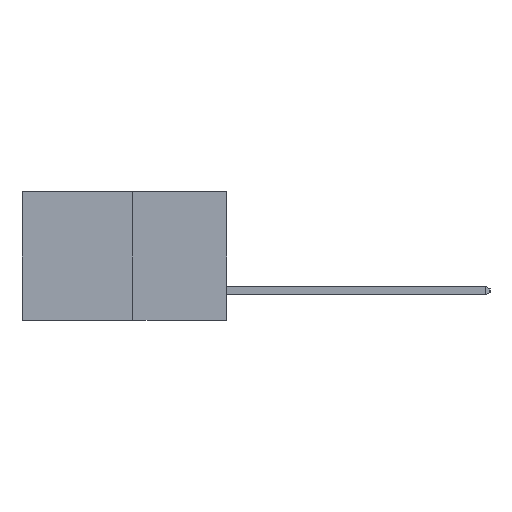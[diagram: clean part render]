
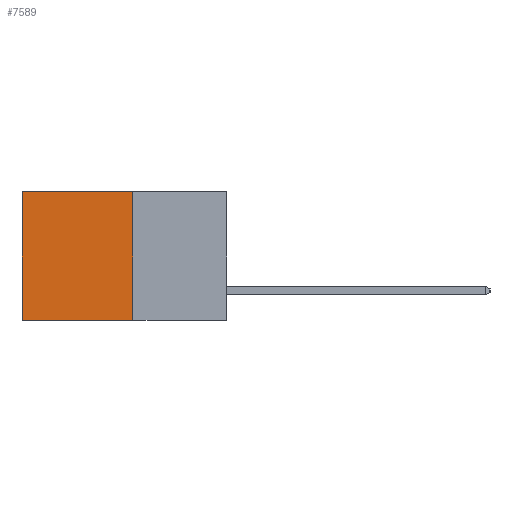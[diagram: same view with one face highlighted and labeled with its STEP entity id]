
A CAD part, left-side view. The second image highlights one B-rep face of the part: STEP entity #7589.
In plain terms, the highlighted planar face has unit normal (-1, 0, 0).
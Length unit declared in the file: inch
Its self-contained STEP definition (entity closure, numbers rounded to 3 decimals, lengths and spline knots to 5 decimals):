
#1554 = ORIENTED_EDGE ( 'NONE', *, *, #25390, .F. ) ;
#1602 = LINE ( 'NONE', #11401, #25249 ) ;
#2268 = DIRECTION ( 'NONE',  ( 0., 1., 0. ) ) ;
#2452 = LINE ( 'NONE', #26547, #19354 ) ;
#2923 = ORIENTED_EDGE ( 'NONE', *, *, #23593, .T. ) ;
#3297 = VECTOR ( 'NONE', #20786, 39.37008 ) ;
#4726 = CARTESIAN_POINT ( 'NONE',  ( 0.277, 0.27, -0.37 ) ) ;
#6753 = CARTESIAN_POINT ( 'NONE',  ( 0.277, 0.27, -0.37 ) ) ;
#6892 = EDGE_CURVE ( 'NONE', #8813, #24257, #26915, .T. ) ;
#7219 = DIRECTION ( 'NONE',  ( 1., 0., 0. ) ) ;
#7589 = ADVANCED_FACE ( 'NONE', ( #12960 ), #16324, .F. ) ;
#8622 = EDGE_CURVE ( 'NONE', #26761, #24257, #2452, .T. ) ;
#8641 = VECTOR ( 'NONE', #15870, 39.37008 ) ;
#8813 = VERTEX_POINT ( 'NONE', #6753 ) ;
#9423 = CARTESIAN_POINT ( 'NONE',  ( 0.277, 0.59, -0.37 ) ) ;
#11401 = CARTESIAN_POINT ( 'NONE',  ( 0.277, 0.27, 0. ) ) ;
#12960 = FACE_OUTER_BOUND ( 'NONE', #13958, .T. ) ;
#13561 = CARTESIAN_POINT ( 'NONE',  ( 0.277, 0.27, -0.37 ) ) ;
#13958 = EDGE_LOOP ( 'NONE', ( #28741, #29041, #1554, #2923 ) ) ;
#15870 = DIRECTION ( 'NONE',  ( 0., 0., -1. ) ) ;
#16324 = PLANE ( 'NONE',  #18593 ) ;
#18593 = AXIS2_PLACEMENT_3D ( 'NONE', #20941, #7219, #23233 ) ;
#19354 = VECTOR ( 'NONE', #24378, 39.37008 ) ;
#20786 = DIRECTION ( 'NONE',  ( 0., 1., 0. ) ) ;
#20854 = LINE ( 'NONE', #13561, #8641 ) ;
#20941 = CARTESIAN_POINT ( 'NONE',  ( 0.277, 0.27, -0.37 ) ) ;
#22909 = CARTESIAN_POINT ( 'NONE',  ( 0.277, 0.27, 0. ) ) ;
#23233 = DIRECTION ( 'NONE',  ( 0., 0., -1. ) ) ;
#23593 = EDGE_CURVE ( 'NONE', #24866, #26761, #1602, .T. ) ;
#24257 = VERTEX_POINT ( 'NONE', #9423 ) ;
#24378 = DIRECTION ( 'NONE',  ( 0., 0., -1. ) ) ;
#24866 = VERTEX_POINT ( 'NONE', #22909 ) ;
#25249 = VECTOR ( 'NONE', #2268, 39.37008 ) ;
#25390 = EDGE_CURVE ( 'NONE', #24866, #8813, #20854, .T. ) ;
#26547 = CARTESIAN_POINT ( 'NONE',  ( 0.277, 0.59, -0.37 ) ) ;
#26761 = VERTEX_POINT ( 'NONE', #27625 ) ;
#26915 = LINE ( 'NONE', #4726, #3297 ) ;
#27625 = CARTESIAN_POINT ( 'NONE',  ( 0.277, 0.59, 0. ) ) ;
#28741 = ORIENTED_EDGE ( 'NONE', *, *, #8622, .T. ) ;
#29041 = ORIENTED_EDGE ( 'NONE', *, *, #6892, .F. ) ;
